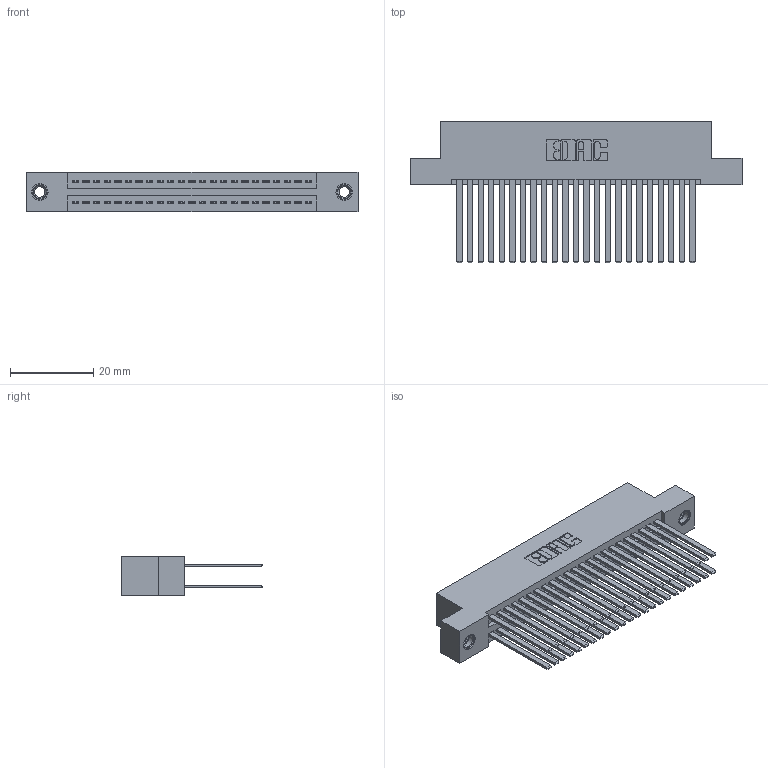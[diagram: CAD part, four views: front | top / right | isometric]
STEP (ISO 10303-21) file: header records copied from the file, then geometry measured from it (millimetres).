
FILE_DESCRIPTION (( 'STEP AP203' ), '1' );
FILE_NAME ('395-046-544-207.STEP', '2019-10-19T04:14:59', ( '' ), ( '' ), 'SwSTEP 2.0', 'SolidWorks 2016', '' );
FILE_SCHEMA (( 'CONFIG_CONTROL_DESIGN' ));
Length unit declared in the file: inch
Products named in the file (4): 345 Part_Flush Mounting Lugs - 0.156 Dia-TI; 345-292-001_345-293-144; 345-250-001_345-250-005-103; 395-046-544-207
Assembly tree (49 placements, depth 2):
  395-046-544-207
    345 Part_Flush Mounting Lugs - 0.156 Dia-TI
    345-292-001_345-293-144  x46
    345-250-001_345-250-005-103  x2
Bounding box: 79.63 x 33.96 x 9.4 mm (x, y, z)
Volume: 8190.2 mm3; surface area: 13656.3 mm2
Topology: 49 solids, 49 shells, 2210 faces, 6503 edges, 4266 vertices
Faces by surface type: plane 1446, cylinder 748, cone 12, torus 4
Entity records: 21606 total; most frequent: CARTESIAN_POINT 3619, ORIENTED_EDGE 3546, DIRECTION 3239, EDGE_CURVE 1773, VECTOR 1533, LINE 1533, VERTEX_POINT 1176, AXIS2_PLACEMENT_3D 853
